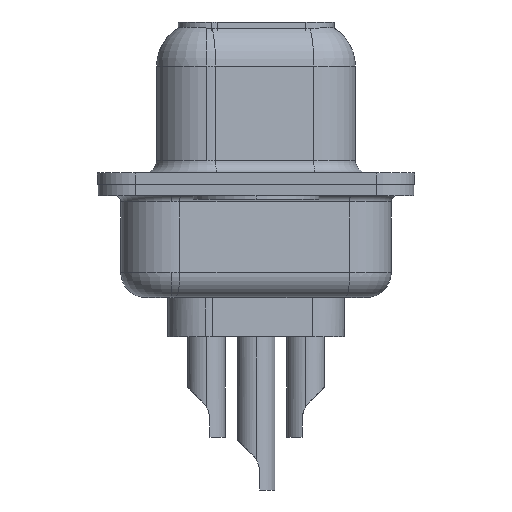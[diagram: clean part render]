
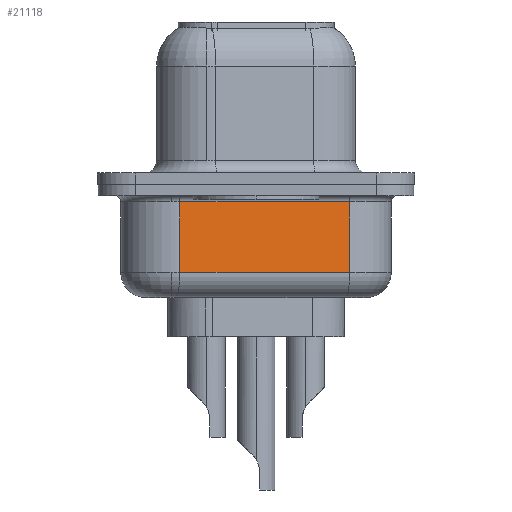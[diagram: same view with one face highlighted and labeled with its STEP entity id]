
A CAD part, left-side view. The second image highlights one B-rep face of the part: STEP entity #21118.
In plain terms, the highlighted planar face has unit normal (-0.985, -0.174, 0).
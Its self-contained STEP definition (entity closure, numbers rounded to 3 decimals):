
#187 = LINE ( 'NONE', #18724, #9531 ) ;
#480 = PLANE ( 'NONE',  #1550 ) ;
#577 = CARTESIAN_POINT ( 'NONE',  ( 4.116, -3.722, -4.5 ) ) ;
#731 = FACE_OUTER_BOUND ( 'NONE', #5273, .T. ) ;
#1116 = VECTOR ( 'NONE', #5991, 1000. ) ;
#1550 = AXIS2_PLACEMENT_3D ( 'NONE', #14566, #19899, #9293 ) ;
#4493 = EDGE_CURVE ( 'NONE', #21487, #10159, #22138, .T. ) ;
#5273 = EDGE_LOOP ( 'NONE', ( #19047, #17455, #8151, #8178 ) ) ;
#5991 = DIRECTION ( 'NONE',  ( 0., 0., 1. ) ) ;
#6601 = DIRECTION ( 'NONE',  ( 0.174, -0.985, 0. ) ) ;
#7642 = CARTESIAN_POINT ( 'NONE',  ( 2.925, 3.028, -4.5 ) ) ;
#7659 = CARTESIAN_POINT ( 'NONE',  ( 2.925, 3.028, -3.5 ) ) ;
#8099 = DIRECTION ( 'NONE',  ( -0.174, 0.985, 0. ) ) ;
#8151 = ORIENTED_EDGE ( 'NONE', *, *, #21778, .T. ) ;
#8178 = ORIENTED_EDGE ( 'NONE', *, *, #15142, .T. ) ;
#8716 = CARTESIAN_POINT ( 'NONE',  ( 2.925, 3.028, -3.5 ) ) ;
#9293 = DIRECTION ( 'NONE',  ( -0.174, 0.985, 0. ) ) ;
#9424 = VERTEX_POINT ( 'NONE', #14539 ) ;
#9501 = EDGE_CURVE ( 'NONE', #21487, #22258, #19862, .T. ) ;
#9531 = VECTOR ( 'NONE', #8099, 1000. ) ;
#10108 = CARTESIAN_POINT ( 'NONE',  ( 4.116, -3.722, -3.5 ) ) ;
#10159 = VERTEX_POINT ( 'NONE', #10108 ) ;
#11610 = VECTOR ( 'NONE', #6601, 1000. ) ;
#12497 = LINE ( 'NONE', #577, #21927 ) ;
#12870 = DIRECTION ( 'NONE',  ( 0., 0., 1. ) ) ;
#14539 = CARTESIAN_POINT ( 'NONE',  ( 4.116, -3.722, -0.7 ) ) ;
#14566 = CARTESIAN_POINT ( 'NONE',  ( 2.925, 3.028, -4.5 ) ) ;
#15142 = EDGE_CURVE ( 'NONE', #9424, #22258, #187, .T. ) ;
#17455 = ORIENTED_EDGE ( 'NONE', *, *, #4493, .T. ) ;
#18724 = CARTESIAN_POINT ( 'NONE',  ( 2.925, 3.028, -0.7 ) ) ;
#19047 = ORIENTED_EDGE ( 'NONE', *, *, #9501, .F. ) ;
#19585 = CARTESIAN_POINT ( 'NONE',  ( 2.925, 3.028, -0.7 ) ) ;
#19862 = LINE ( 'NONE', #7642, #1116 ) ;
#19899 = DIRECTION ( 'NONE',  ( 0.985, 0.174, 0. ) ) ;
#21118 = ADVANCED_FACE ( 'NONE', ( #731 ), #480, .F. ) ;
#21487 = VERTEX_POINT ( 'NONE', #8716 ) ;
#21778 = EDGE_CURVE ( 'NONE', #10159, #9424, #12497, .T. ) ;
#21927 = VECTOR ( 'NONE', #12870, 1000. ) ;
#22138 = LINE ( 'NONE', #7659, #11610 ) ;
#22258 = VERTEX_POINT ( 'NONE', #19585 ) ;
